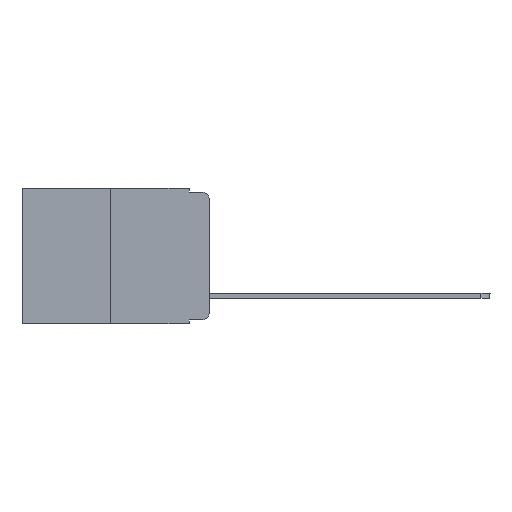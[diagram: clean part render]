
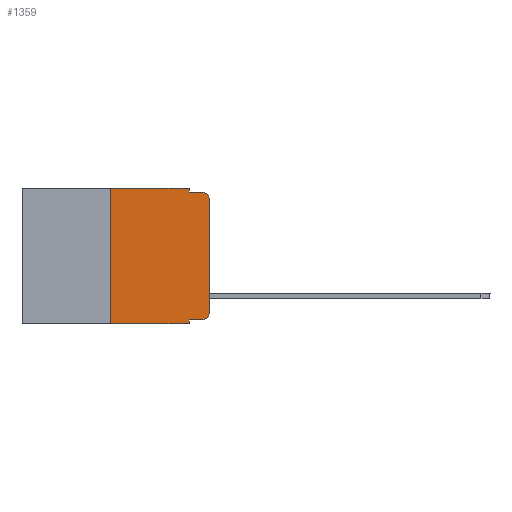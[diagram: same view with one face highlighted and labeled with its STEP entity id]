
A CAD part, left-side view. The second image highlights one B-rep face of the part: STEP entity #1359.
In plain terms, the highlighted planar face has unit normal (-1, 0, 0).
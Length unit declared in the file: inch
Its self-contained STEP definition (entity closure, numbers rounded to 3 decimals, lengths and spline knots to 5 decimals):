
#729 = EDGE_CURVE ( 'NONE', #6791, #17240, #6576, .T. ) ;
#777 = ORIENTED_EDGE ( 'NONE', *, *, #729, .F. ) ;
#826 = EDGE_CURVE ( 'NONE', #3037, #17719, #5583, .T. ) ;
#1359 = ADVANCED_FACE ( 'NONE', ( #5025 ), #5320, .F. ) ;
#1525 = CARTESIAN_POINT ( 'NONE',  ( 0., 0.051, 0. ) ) ;
#1740 = VERTEX_POINT ( 'NONE', #13038 ) ;
#2091 = CARTESIAN_POINT ( 'NONE',  ( 0., 0., 0. ) ) ;
#2149 = DIRECTION ( 'NONE',  ( 0., 0., -1. ) ) ;
#2154 = DIRECTION ( 'NONE',  ( 0., 0., 1. ) ) ;
#2298 = CIRCLE ( 'NONE', #15393, 0.02 ) ;
#2426 = VECTOR ( 'NONE', #6390, 39.37008 ) ;
#2635 = EDGE_CURVE ( 'NONE', #5355, #3037, #2298, .T. ) ;
#2716 = VERTEX_POINT ( 'NONE', #16918 ) ;
#3037 = VERTEX_POINT ( 'NONE', #3098 ) ;
#3048 = DIRECTION ( 'NONE',  ( 0., -1., 0. ) ) ;
#3098 = CARTESIAN_POINT ( 'NONE',  ( 0., 0., -0.313 ) ) ;
#3323 = LINE ( 'NONE', #19045, #15405 ) ;
#3374 = CARTESIAN_POINT ( 'NONE',  ( 0., 0.051, 0. ) ) ;
#3549 = VERTEX_POINT ( 'NONE', #16658 ) ;
#4107 = CARTESIAN_POINT ( 'NONE',  ( 0., 0.02, -0.313 ) ) ;
#4284 = CARTESIAN_POINT ( 'NONE',  ( 0., 0.473, -0.343 ) ) ;
#4493 = ORIENTED_EDGE ( 'NONE', *, *, #6242, .T. ) ;
#5025 = FACE_OUTER_BOUND ( 'NONE', #9162, .T. ) ;
#5320 = PLANE ( 'NONE',  #19250 ) ;
#5347 = DIRECTION ( 'NONE',  ( 0., 0., 1. ) ) ;
#5355 = VERTEX_POINT ( 'NONE', #18686 ) ;
#5583 = LINE ( 'NONE', #2091, #7311 ) ;
#5720 = ORIENTED_EDGE ( 'NONE', *, *, #6429, .F. ) ;
#6242 = EDGE_CURVE ( 'NONE', #1740, #5355, #11247, .T. ) ;
#6275 = VECTOR ( 'NONE', #5347, 39.37008 ) ;
#6327 = LINE ( 'NONE', #1525, #14233 ) ;
#6390 = DIRECTION ( 'NONE',  ( 0., 0., -1. ) ) ;
#6394 = DIRECTION ( 'NONE',  ( 0., -1., 0. ) ) ;
#6429 = EDGE_CURVE ( 'NONE', #2716, #7744, #9513, .T. ) ;
#6453 = CARTESIAN_POINT ( 'NONE',  ( 0., 0.051, -0.01 ) ) ;
#6486 = CIRCLE ( 'NONE', #10402, 0.02 ) ;
#6523 = LINE ( 'NONE', #6453, #16402 ) ;
#6576 = LINE ( 'NONE', #3374, #2426 ) ;
#6715 = ORIENTED_EDGE ( 'NONE', *, *, #9483, .T. ) ;
#6791 = VERTEX_POINT ( 'NONE', #18675 ) ;
#7311 = VECTOR ( 'NONE', #2154, 39.37008 ) ;
#7744 = VERTEX_POINT ( 'NONE', #17287 ) ;
#8405 = VERTEX_POINT ( 'NONE', #18837 ) ;
#8460 = EDGE_CURVE ( 'NONE', #17240, #3549, #6523, .T. ) ;
#9016 = DIRECTION ( 'NONE',  ( 0., 0., -1. ) ) ;
#9162 = EDGE_LOOP ( 'NONE', ( #12681, #6715, #16431, #777, #18192, #5720, #10269, #15348, #4493, #9957 ) ) ;
#9479 = EDGE_CURVE ( 'NONE', #2716, #8405, #16112, .T. ) ;
#9483 = EDGE_CURVE ( 'NONE', #17719, #3549, #6486, .T. ) ;
#9513 = LINE ( 'NONE', #14802, #6275 ) ;
#9957 = ORIENTED_EDGE ( 'NONE', *, *, #2635, .T. ) ;
#10219 = VECTOR ( 'NONE', #16887, 39.37008 ) ;
#10269 = ORIENTED_EDGE ( 'NONE', *, *, #9479, .T. ) ;
#10402 = AXIS2_PLACEMENT_3D ( 'NONE', #19955, #18519, #13868 ) ;
#11247 = LINE ( 'NONE', #12882, #14433 ) ;
#11900 = DIRECTION ( 'NONE',  ( 0., 0., -1. ) ) ;
#12681 = ORIENTED_EDGE ( 'NONE', *, *, #826, .T. ) ;
#12882 = CARTESIAN_POINT ( 'NONE',  ( 0., 0.051, -0.333 ) ) ;
#13038 = CARTESIAN_POINT ( 'NONE',  ( 0., 0.051, -0.333 ) ) ;
#13382 = EDGE_CURVE ( 'NONE', #1740, #8405, #6327, .T. ) ;
#13868 = DIRECTION ( 'NONE',  ( 0., 0., -1. ) ) ;
#14233 = VECTOR ( 'NONE', #2149, 39.37008 ) ;
#14433 = VECTOR ( 'NONE', #6394, 39.37008 ) ;
#14802 = CARTESIAN_POINT ( 'NONE',  ( 0., 0.25, 0. ) ) ;
#15348 = ORIENTED_EDGE ( 'NONE', *, *, #13382, .F. ) ;
#15393 = AXIS2_PLACEMENT_3D ( 'NONE', #4107, #19983, #9016 ) ;
#15405 = VECTOR ( 'NONE', #15859, 39.37008 ) ;
#15859 = DIRECTION ( 'NONE',  ( 0., -1., 0. ) ) ;
#15989 = EDGE_CURVE ( 'NONE', #7744, #6791, #3323, .T. ) ;
#16112 = LINE ( 'NONE', #4284, #10219 ) ;
#16402 = VECTOR ( 'NONE', #3048, 39.37008 ) ;
#16431 = ORIENTED_EDGE ( 'NONE', *, *, #8460, .F. ) ;
#16658 = CARTESIAN_POINT ( 'NONE',  ( 0., 0.02, -0.01 ) ) ;
#16887 = DIRECTION ( 'NONE',  ( 0., -1., 0. ) ) ;
#16918 = CARTESIAN_POINT ( 'NONE',  ( 0., 0.25, -0.343 ) ) ;
#17240 = VERTEX_POINT ( 'NONE', #18818 ) ;
#17287 = CARTESIAN_POINT ( 'NONE',  ( 0., 0.25, 0. ) ) ;
#17719 = VERTEX_POINT ( 'NONE', #18946 ) ;
#18120 = CARTESIAN_POINT ( 'NONE',  ( 0., 0.473, 0. ) ) ;
#18192 = ORIENTED_EDGE ( 'NONE', *, *, #15989, .F. ) ;
#18195 = DIRECTION ( 'NONE',  ( 1., 0., 0. ) ) ;
#18519 = DIRECTION ( 'NONE',  ( -1., 0., 0. ) ) ;
#18675 = CARTESIAN_POINT ( 'NONE',  ( 0., 0.051, 0. ) ) ;
#18686 = CARTESIAN_POINT ( 'NONE',  ( 0., 0.02, -0.333 ) ) ;
#18818 = CARTESIAN_POINT ( 'NONE',  ( 0., 0.051, -0.01 ) ) ;
#18837 = CARTESIAN_POINT ( 'NONE',  ( 0., 0.051, -0.343 ) ) ;
#18946 = CARTESIAN_POINT ( 'NONE',  ( 0., 0., -0.03 ) ) ;
#19045 = CARTESIAN_POINT ( 'NONE',  ( 0., 0.473, 0. ) ) ;
#19250 = AXIS2_PLACEMENT_3D ( 'NONE', #18120, #18195, #11900 ) ;
#19955 = CARTESIAN_POINT ( 'NONE',  ( 0., 0.02, -0.03 ) ) ;
#19983 = DIRECTION ( 'NONE',  ( -1., 0., 0. ) ) ;
